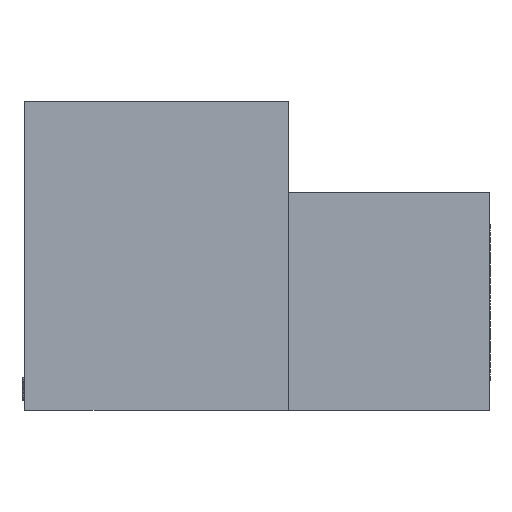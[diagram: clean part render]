
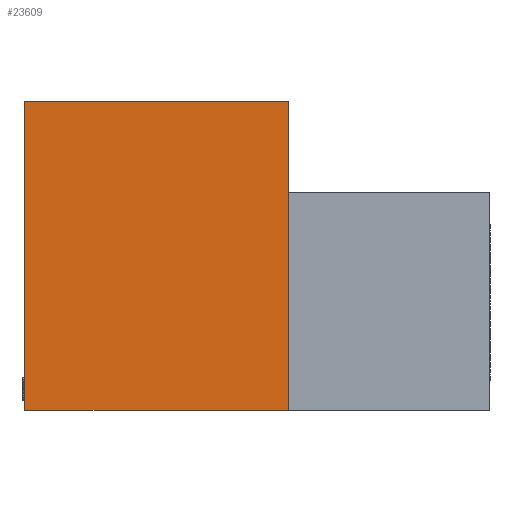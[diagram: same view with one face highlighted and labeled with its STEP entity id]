
A CAD part, left-side view. The second image highlights one B-rep face of the part: STEP entity #23609.
In plain terms, the highlighted planar face has unit normal (-1, 0, 0).
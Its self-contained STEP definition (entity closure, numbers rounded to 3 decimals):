
#1988 = VERTEX_POINT ( 'NONE', #15079 ) ;
#2143 = CARTESIAN_POINT ( 'NONE',  ( 0., 11.506, 0. ) ) ;
#2466 = VECTOR ( 'NONE', #15414, 1000. ) ;
#3989 = DIRECTION ( 'NONE',  ( 1., 0., 0. ) ) ;
#4228 = CARTESIAN_POINT ( 'NONE',  ( 0., 11.506, 0. ) ) ;
#5418 = DIRECTION ( 'NONE',  ( 0., -1., 0. ) ) ;
#5636 = CARTESIAN_POINT ( 'NONE',  ( 0., 11.506, -13.487 ) ) ;
#7941 = EDGE_CURVE ( 'NONE', #1988, #34027, #32280, .T. ) ;
#8698 = EDGE_CURVE ( 'NONE', #22329, #12453, #40250, .T. ) ;
#9005 = CARTESIAN_POINT ( 'NONE',  ( 0., 0., -13.487 ) ) ;
#10549 = ORIENTED_EDGE ( 'NONE', *, *, #8698, .F. ) ;
#10780 = FACE_OUTER_BOUND ( 'NONE', #26541, .T. ) ;
#11136 = ORIENTED_EDGE ( 'NONE', *, *, #22826, .F. ) ;
#12453 = VERTEX_POINT ( 'NONE', #4228 ) ;
#14261 = LINE ( 'NONE', #2143, #21334 ) ;
#14327 = DIRECTION ( 'NONE',  ( 0., 1., 0. ) ) ;
#15079 = CARTESIAN_POINT ( 'NONE',  ( 0., 0., 0. ) ) ;
#15414 = DIRECTION ( 'NONE',  ( 0., 0., 1. ) ) ;
#15438 = VECTOR ( 'NONE', #14327, 1000. ) ;
#16894 = PLANE ( 'NONE',  #31670 ) ;
#17859 = EDGE_CURVE ( 'NONE', #34027, #22329, #24496, .T. ) ;
#18275 = ORIENTED_EDGE ( 'NONE', *, *, #17859, .F. ) ;
#20536 = CARTESIAN_POINT ( 'NONE',  ( 0., 0., 0. ) ) ;
#21334 = VECTOR ( 'NONE', #5418, 1000. ) ;
#22329 = VERTEX_POINT ( 'NONE', #28958 ) ;
#22826 = EDGE_CURVE ( 'NONE', #12453, #1988, #14261, .T. ) ;
#23609 = ADVANCED_FACE ( 'NONE', ( #10780 ), #16894, .F. ) ;
#24496 = LINE ( 'NONE', #30425, #15438 ) ;
#26541 = EDGE_LOOP ( 'NONE', ( #18275, #34658, #11136, #10549 ) ) ;
#28958 = CARTESIAN_POINT ( 'NONE',  ( 0., 11.506, -13.487 ) ) ;
#29608 = DIRECTION ( 'NONE',  ( 0., 0., -1. ) ) ;
#30425 = CARTESIAN_POINT ( 'NONE',  ( 0., -8.814, -13.487 ) ) ;
#31670 = AXIS2_PLACEMENT_3D ( 'NONE', #36345, #3989, #36072 ) ;
#31823 = VECTOR ( 'NONE', #29608, 1000. ) ;
#32280 = LINE ( 'NONE', #20536, #31823 ) ;
#34027 = VERTEX_POINT ( 'NONE', #9005 ) ;
#34658 = ORIENTED_EDGE ( 'NONE', *, *, #7941, .F. ) ;
#36072 = DIRECTION ( 'NONE',  ( 0., 0., -1. ) ) ;
#36345 = CARTESIAN_POINT ( 'NONE',  ( 0., 0., 0. ) ) ;
#40250 = LINE ( 'NONE', #5636, #2466 ) ;
